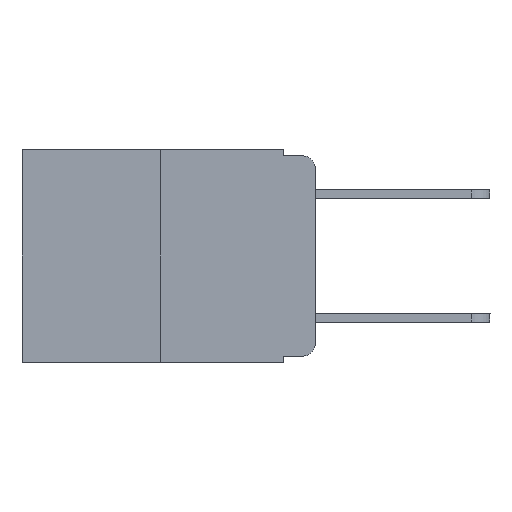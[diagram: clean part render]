
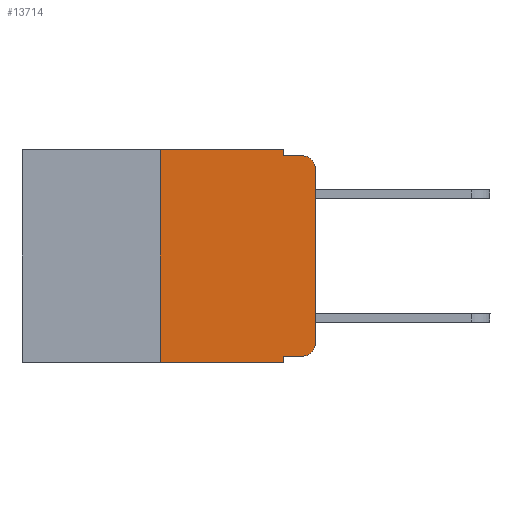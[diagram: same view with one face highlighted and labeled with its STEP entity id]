
A CAD part, left-side view. The second image highlights one B-rep face of the part: STEP entity #13714.
In plain terms, the highlighted planar face has unit normal (-1, 0, 0).
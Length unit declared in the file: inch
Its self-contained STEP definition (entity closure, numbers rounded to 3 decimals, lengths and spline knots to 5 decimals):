
#151 = EDGE_CURVE ( 'NONE', #19606, #6611, #334, .T. ) ;
#334 = LINE ( 'NONE', #14496, #7213 ) ;
#528 = VERTEX_POINT ( 'NONE', #6870 ) ;
#982 = DIRECTION ( 'NONE',  ( 0., 0., -1. ) ) ;
#1035 = VECTOR ( 'NONE', #10058, 39.37008 ) ;
#1365 = ORIENTED_EDGE ( 'NONE', *, *, #7725, .F. ) ;
#1582 = LINE ( 'NONE', #3273, #1035 ) ;
#1725 = DIRECTION ( 'NONE',  ( 0., -1., 0. ) ) ;
#2460 = DIRECTION ( 'NONE',  ( 0., -1., 0. ) ) ;
#2473 = EDGE_CURVE ( 'NONE', #17192, #5715, #14810, .T. ) ;
#2580 = DIRECTION ( 'NONE',  ( 0., 0., -1. ) ) ;
#2664 = CARTESIAN_POINT ( 'NONE',  ( 0., 0.051, 0. ) ) ;
#2715 = ORIENTED_EDGE ( 'NONE', *, *, #2473, .F. ) ;
#3119 = CARTESIAN_POINT ( 'NONE',  ( 0., 0.473, 0. ) ) ;
#3273 = CARTESIAN_POINT ( 'NONE',  ( 0., 0.25, 0. ) ) ;
#3402 = ORIENTED_EDGE ( 'NONE', *, *, #4557, .T. ) ;
#4272 = LINE ( 'NONE', #4313, #19135 ) ;
#4276 = CARTESIAN_POINT ( 'NONE',  ( 0., 0.473, -0.343 ) ) ;
#4313 = CARTESIAN_POINT ( 'NONE',  ( 0., 0.051, -0.333 ) ) ;
#4432 = LINE ( 'NONE', #14081, #16799 ) ;
#4557 = EDGE_CURVE ( 'NONE', #17192, #18797, #4272, .T. ) ;
#5457 = CARTESIAN_POINT ( 'NONE',  ( 0., 0.051, -0.333 ) ) ;
#5477 = EDGE_LOOP ( 'NONE', ( #7095, #10584, #11781, #1365, #17486, #18105, #20482, #2715, #3402, #19644 ) ) ;
#5715 = VERTEX_POINT ( 'NONE', #17556 ) ;
#6267 = VECTOR ( 'NONE', #17252, 39.37008 ) ;
#6280 = PLANE ( 'NONE',  #13493 ) ;
#6611 = VERTEX_POINT ( 'NONE', #11025 ) ;
#6870 = CARTESIAN_POINT ( 'NONE',  ( 0., 0.051, 0. ) ) ;
#7095 = ORIENTED_EDGE ( 'NONE', *, *, #151, .T. ) ;
#7213 = VECTOR ( 'NONE', #19939, 39.37008 ) ;
#7249 = DIRECTION ( 'NONE',  ( 0., 0., -1. ) ) ;
#7521 = EDGE_CURVE ( 'NONE', #18797, #19606, #20428, .T. ) ;
#7543 = VERTEX_POINT ( 'NONE', #13331 ) ;
#7725 = EDGE_CURVE ( 'NONE', #528, #18095, #4432, .T. ) ;
#7740 = DIRECTION ( 'NONE',  ( 0., -1., 0. ) ) ;
#8611 = DIRECTION ( 'NONE',  ( -1., 0., 0. ) ) ;
#8839 = DIRECTION ( 'NONE',  ( 0., 0., -1. ) ) ;
#9324 = VERTEX_POINT ( 'NONE', #14667 ) ;
#9761 = EDGE_CURVE ( 'NONE', #6611, #13108, #14776, .T. ) ;
#9866 = VECTOR ( 'NONE', #7740, 39.37008 ) ;
#10058 = DIRECTION ( 'NONE',  ( 0., 0., 1. ) ) ;
#10242 = CARTESIAN_POINT ( 'NONE',  ( 0., 0.051, -0.01 ) ) ;
#10339 = EDGE_CURVE ( 'NONE', #18095, #13108, #22208, .T. ) ;
#10466 = CARTESIAN_POINT ( 'NONE',  ( 0., 0.02, -0.03 ) ) ;
#10584 = ORIENTED_EDGE ( 'NONE', *, *, #9761, .T. ) ;
#11025 = CARTESIAN_POINT ( 'NONE',  ( 0., 0., -0.03 ) ) ;
#11530 = DIRECTION ( 'NONE',  ( 1., 0., 0. ) ) ;
#11570 = DIRECTION ( 'NONE',  ( -1., 0., 0. ) ) ;
#11781 = ORIENTED_EDGE ( 'NONE', *, *, #10339, .F. ) ;
#13108 = VERTEX_POINT ( 'NONE', #13242 ) ;
#13151 = LINE ( 'NONE', #4276, #9866 ) ;
#13242 = CARTESIAN_POINT ( 'NONE',  ( 0., 0.02, -0.01 ) ) ;
#13331 = CARTESIAN_POINT ( 'NONE',  ( 0., 0.25, -0.343 ) ) ;
#13432 = CARTESIAN_POINT ( 'NONE',  ( 0., 0.02, -0.333 ) ) ;
#13493 = AXIS2_PLACEMENT_3D ( 'NONE', #18357, #11530, #982 ) ;
#13714 = ADVANCED_FACE ( 'NONE', ( #16610 ), #6280, .F. ) ;
#13781 = DIRECTION ( 'NONE',  ( 0., 0., -1. ) ) ;
#14081 = CARTESIAN_POINT ( 'NONE',  ( 0., 0.051, 0. ) ) ;
#14496 = CARTESIAN_POINT ( 'NONE',  ( 0., 0., 0. ) ) ;
#14536 = CARTESIAN_POINT ( 'NONE',  ( 0., 0., -0.313 ) ) ;
#14667 = CARTESIAN_POINT ( 'NONE',  ( 0., 0.25, 0. ) ) ;
#14776 = CIRCLE ( 'NONE', #17412, 0.02 ) ;
#14810 = LINE ( 'NONE', #2664, #22552 ) ;
#15465 = CARTESIAN_POINT ( 'NONE',  ( 0., 0.02, -0.313 ) ) ;
#16610 = FACE_OUTER_BOUND ( 'NONE', #5477, .T. ) ;
#16799 = VECTOR ( 'NONE', #7249, 39.37008 ) ;
#17192 = VERTEX_POINT ( 'NONE', #5457 ) ;
#17250 = AXIS2_PLACEMENT_3D ( 'NONE', #15465, #11570, #13781 ) ;
#17252 = DIRECTION ( 'NONE',  ( 0., -1., 0. ) ) ;
#17412 = AXIS2_PLACEMENT_3D ( 'NONE', #10466, #8611, #8839 ) ;
#17484 = VECTOR ( 'NONE', #1725, 39.37008 ) ;
#17486 = ORIENTED_EDGE ( 'NONE', *, *, #18822, .F. ) ;
#17556 = CARTESIAN_POINT ( 'NONE',  ( 0., 0.051, -0.343 ) ) ;
#18095 = VERTEX_POINT ( 'NONE', #10242 ) ;
#18105 = ORIENTED_EDGE ( 'NONE', *, *, #18829, .F. ) ;
#18357 = CARTESIAN_POINT ( 'NONE',  ( 0., 0.473, 0. ) ) ;
#18797 = VERTEX_POINT ( 'NONE', #13432 ) ;
#18822 = EDGE_CURVE ( 'NONE', #9324, #528, #20313, .T. ) ;
#18829 = EDGE_CURVE ( 'NONE', #7543, #9324, #1582, .T. ) ;
#19135 = VECTOR ( 'NONE', #2460, 39.37008 ) ;
#19606 = VERTEX_POINT ( 'NONE', #14536 ) ;
#19644 = ORIENTED_EDGE ( 'NONE', *, *, #7521, .T. ) ;
#19939 = DIRECTION ( 'NONE',  ( 0., 0., 1. ) ) ;
#20313 = LINE ( 'NONE', #3119, #6267 ) ;
#20428 = CIRCLE ( 'NONE', #17250, 0.02 ) ;
#20482 = ORIENTED_EDGE ( 'NONE', *, *, #20513, .T. ) ;
#20513 = EDGE_CURVE ( 'NONE', #7543, #5715, #13151, .T. ) ;
#21124 = CARTESIAN_POINT ( 'NONE',  ( 0., 0.051, -0.01 ) ) ;
#22208 = LINE ( 'NONE', #21124, #17484 ) ;
#22552 = VECTOR ( 'NONE', #2580, 39.37008 ) ;
